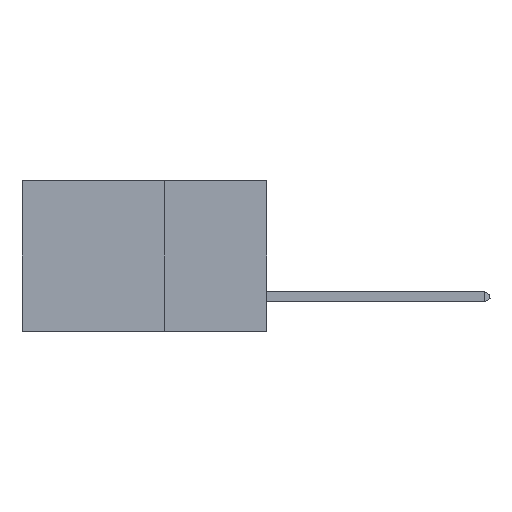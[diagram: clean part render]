
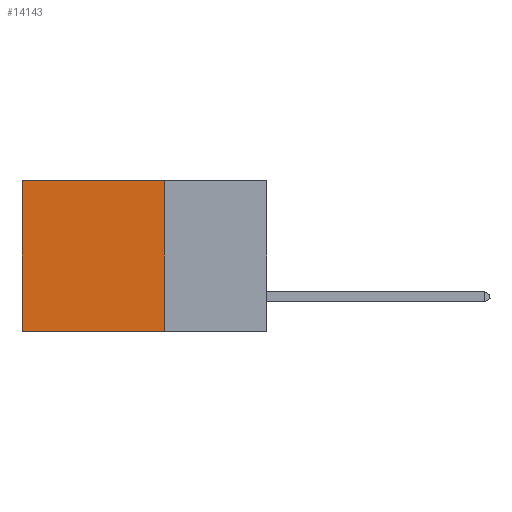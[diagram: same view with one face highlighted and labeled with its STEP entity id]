
A CAD part, left-side view. The second image highlights one B-rep face of the part: STEP entity #14143.
In plain terms, the highlighted planar face has unit normal (-1, 0, 0).
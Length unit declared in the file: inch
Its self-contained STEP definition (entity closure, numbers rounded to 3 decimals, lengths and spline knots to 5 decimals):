
#126 = EDGE_CURVE ( 'NONE', #9871, #14524, #12433, .T. ) ;
#618 = CARTESIAN_POINT ( 'NONE',  ( 0.2875, 0.25, -0.37 ) ) ;
#677 = CARTESIAN_POINT ( 'NONE',  ( 0.2875, 0.6, 0. ) ) ;
#900 = VECTOR ( 'NONE', #6524, 39.37008 ) ;
#962 = VERTEX_POINT ( 'NONE', #6256 ) ;
#1114 = DIRECTION ( 'NONE',  ( 0., 0., -1. ) ) ;
#1168 = DIRECTION ( 'NONE',  ( 1., 0., 0. ) ) ;
#1992 = EDGE_CURVE ( 'NONE', #962, #3872, #14048, .T. ) ;
#2754 = VECTOR ( 'NONE', #11817, 39.37008 ) ;
#3797 = VECTOR ( 'NONE', #10901, 39.37008 ) ;
#3872 = VERTEX_POINT ( 'NONE', #618 ) ;
#4217 = EDGE_LOOP ( 'NONE', ( #7942, #7801, #12069, #10467 ) ) ;
#4597 = CARTESIAN_POINT ( 'NONE',  ( 0.2875, 0.25, 0. ) ) ;
#4690 = CARTESIAN_POINT ( 'NONE',  ( 0.2875, 0.6, -0.37 ) ) ;
#5377 = CARTESIAN_POINT ( 'NONE',  ( 0.2875, 0.25, 0. ) ) ;
#6256 = CARTESIAN_POINT ( 'NONE',  ( 0.2875, 0.25, 0. ) ) ;
#6315 = VECTOR ( 'NONE', #11559, 39.37008 ) ;
#6524 = DIRECTION ( 'NONE',  ( 0., 1., 0. ) ) ;
#7074 = EDGE_CURVE ( 'NONE', #3872, #14524, #9411, .T. ) ;
#7801 = ORIENTED_EDGE ( 'NONE', *, *, #7074, .F. ) ;
#7942 = ORIENTED_EDGE ( 'NONE', *, *, #126, .T. ) ;
#9411 = LINE ( 'NONE', #12940, #2754 ) ;
#9871 = VERTEX_POINT ( 'NONE', #12627 ) ;
#10429 = CARTESIAN_POINT ( 'NONE',  ( 0.2875, 0.25, 0. ) ) ;
#10467 = ORIENTED_EDGE ( 'NONE', *, *, #14816, .T. ) ;
#10901 = DIRECTION ( 'NONE',  ( 0., 0., -1. ) ) ;
#11316 = PLANE ( 'NONE',  #11526 ) ;
#11526 = AXIS2_PLACEMENT_3D ( 'NONE', #4597, #1168, #1114 ) ;
#11538 = LINE ( 'NONE', #5377, #900 ) ;
#11559 = DIRECTION ( 'NONE',  ( 0., 0., -1. ) ) ;
#11817 = DIRECTION ( 'NONE',  ( 0., 1., 0. ) ) ;
#12069 = ORIENTED_EDGE ( 'NONE', *, *, #1992, .F. ) ;
#12433 = LINE ( 'NONE', #677, #3797 ) ;
#12627 = CARTESIAN_POINT ( 'NONE',  ( 0.2875, 0.6, 0. ) ) ;
#12940 = CARTESIAN_POINT ( 'NONE',  ( 0.2875, 0.25, -0.37 ) ) ;
#14048 = LINE ( 'NONE', #10429, #6315 ) ;
#14143 = ADVANCED_FACE ( 'NONE', ( #14298 ), #11316, .F. ) ;
#14298 = FACE_OUTER_BOUND ( 'NONE', #4217, .T. ) ;
#14524 = VERTEX_POINT ( 'NONE', #4690 ) ;
#14816 = EDGE_CURVE ( 'NONE', #962, #9871, #11538, .T. ) ;
